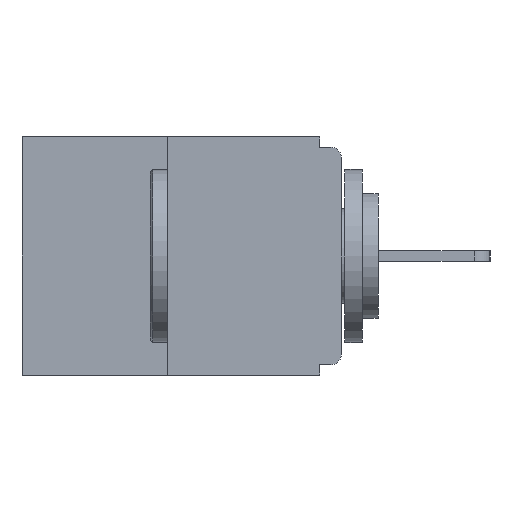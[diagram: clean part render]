
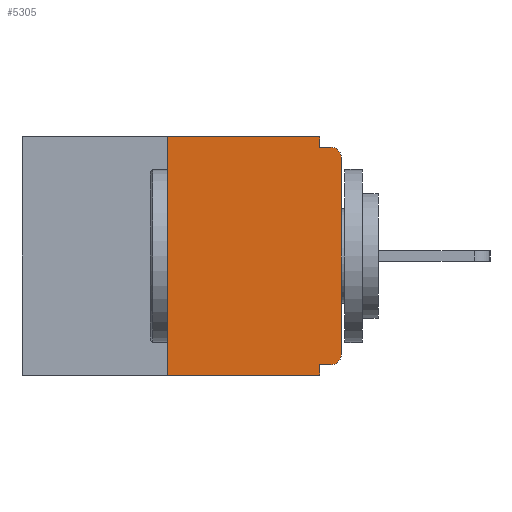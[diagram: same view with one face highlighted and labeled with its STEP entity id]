
A CAD part, left-side view. The second image highlights one B-rep face of the part: STEP entity #5305.
In plain terms, the highlighted planar face has unit normal (-1, 0, 0).
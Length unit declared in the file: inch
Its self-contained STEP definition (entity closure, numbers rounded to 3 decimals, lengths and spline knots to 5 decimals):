
#21 = EDGE_CURVE ( 'NONE', #17906, #2304, #659, .T. ) ;
#180 = ORIENTED_EDGE ( 'NONE', *, *, #4818, .T. ) ;
#387 = CARTESIAN_POINT ( 'NONE',  ( 0., 0.46, 0. ) ) ;
#618 = VECTOR ( 'NONE', #17796, 39.37008 ) ;
#659 = LINE ( 'NONE', #6343, #618 ) ;
#941 = EDGE_LOOP ( 'NONE', ( #14344, #11404, #3829, #10271, #18265, #13380, #5420, #180, #15805, #8281 ) ) ;
#1195 = DIRECTION ( 'NONE',  ( -1., 0., 0. ) ) ;
#1863 = AXIS2_PLACEMENT_3D ( 'NONE', #5914, #3127, #4519 ) ;
#2304 = VERTEX_POINT ( 'NONE', #2717 ) ;
#2305 = CARTESIAN_POINT ( 'NONE',  ( 0., 0.015, -0.328 ) ) ;
#2473 = AXIS2_PLACEMENT_3D ( 'NONE', #387, #11800, #11610 ) ;
#2684 = CARTESIAN_POINT ( 'NONE',  ( 0., 0.031, -0.015 ) ) ;
#2700 = DIRECTION ( 'NONE',  ( 0., 0., 1. ) ) ;
#2717 = CARTESIAN_POINT ( 'NONE',  ( 0., 0., -0.03 ) ) ;
#3127 = DIRECTION ( 'NONE',  ( -1., 0., 0. ) ) ;
#3203 = LINE ( 'NONE', #14530, #13270 ) ;
#3829 = ORIENTED_EDGE ( 'NONE', *, *, #13297, .T. ) ;
#3944 = LINE ( 'NONE', #6741, #12416 ) ;
#4097 = CARTESIAN_POINT ( 'NONE',  ( 0., 0., -0.328 ) ) ;
#4271 = DIRECTION ( 'NONE',  ( 0., 1., 0. ) ) ;
#4519 = DIRECTION ( 'NONE',  ( 0., 0., -1. ) ) ;
#4671 = CARTESIAN_POINT ( 'NONE',  ( 0., 0.031, -0.343 ) ) ;
#4739 = VERTEX_POINT ( 'NONE', #2305 ) ;
#4770 = CARTESIAN_POINT ( 'NONE',  ( 0., 0.25, 0. ) ) ;
#4818 = EDGE_CURVE ( 'NONE', #2304, #14982, #8431, .T. ) ;
#5305 = ADVANCED_FACE ( 'NONE', ( #7473 ), #8697, .F. ) ;
#5420 = ORIENTED_EDGE ( 'NONE', *, *, #21, .T. ) ;
#5493 = LINE ( 'NONE', #4097, #14972 ) ;
#5914 = CARTESIAN_POINT ( 'NONE',  ( 0., 0.015, -0.03 ) ) ;
#6343 = CARTESIAN_POINT ( 'NONE',  ( 0., 0., 0. ) ) ;
#6741 = CARTESIAN_POINT ( 'NONE',  ( 0., 0.46, -0.343 ) ) ;
#6895 = VERTEX_POINT ( 'NONE', #4671 ) ;
#7255 = VECTOR ( 'NONE', #13898, 39.37008 ) ;
#7466 = EDGE_CURVE ( 'NONE', #14918, #6895, #15384, .T. ) ;
#7473 = FACE_OUTER_BOUND ( 'NONE', #941, .T. ) ;
#7769 = EDGE_CURVE ( 'NONE', #10891, #12448, #3203, .T. ) ;
#8281 = ORIENTED_EDGE ( 'NONE', *, *, #18342, .F. ) ;
#8401 = CARTESIAN_POINT ( 'NONE',  ( 0., 0.015, -0.015 ) ) ;
#8431 = CIRCLE ( 'NONE', #1863, 0.015 ) ;
#8697 = PLANE ( 'NONE',  #2473 ) ;
#9292 = CARTESIAN_POINT ( 'NONE',  ( 0., 0., -0.313 ) ) ;
#9453 = CARTESIAN_POINT ( 'NONE',  ( 0., 0.031, 0. ) ) ;
#10120 = DIRECTION ( 'NONE',  ( 0., -1., 0. ) ) ;
#10271 = ORIENTED_EDGE ( 'NONE', *, *, #7466, .F. ) ;
#10651 = CARTESIAN_POINT ( 'NONE',  ( 0., 0.031, 0. ) ) ;
#10891 = VERTEX_POINT ( 'NONE', #4770 ) ;
#10920 = CARTESIAN_POINT ( 'NONE',  ( 0., 0.015, -0.313 ) ) ;
#11103 = VECTOR ( 'NONE', #10120, 39.37008 ) ;
#11116 = EDGE_CURVE ( 'NONE', #17184, #10891, #15722, .T. ) ;
#11152 = VECTOR ( 'NONE', #2700, 39.37008 ) ;
#11404 = ORIENTED_EDGE ( 'NONE', *, *, #11116, .F. ) ;
#11610 = DIRECTION ( 'NONE',  ( 0., 0., -1. ) ) ;
#11616 = DIRECTION ( 'NONE',  ( 0., -1., 0. ) ) ;
#11800 = DIRECTION ( 'NONE',  ( 1., 0., 0. ) ) ;
#12106 = AXIS2_PLACEMENT_3D ( 'NONE', #10920, #1195, #18325 ) ;
#12416 = VECTOR ( 'NONE', #12464, 39.37008 ) ;
#12448 = VERTEX_POINT ( 'NONE', #10651 ) ;
#12464 = DIRECTION ( 'NONE',  ( 0., -1., 0. ) ) ;
#12644 = EDGE_CURVE ( 'NONE', #4739, #17906, #12712, .T. ) ;
#12712 = CIRCLE ( 'NONE', #12106, 0.015 ) ;
#13270 = VECTOR ( 'NONE', #11616, 39.37008 ) ;
#13297 = EDGE_CURVE ( 'NONE', #17184, #6895, #3944, .T. ) ;
#13380 = ORIENTED_EDGE ( 'NONE', *, *, #12644, .T. ) ;
#13482 = LINE ( 'NONE', #9453, #15305 ) ;
#13898 = DIRECTION ( 'NONE',  ( 0., 0., -1. ) ) ;
#13959 = CARTESIAN_POINT ( 'NONE',  ( 0., 0.031, -0.328 ) ) ;
#14344 = ORIENTED_EDGE ( 'NONE', *, *, #7769, .F. ) ;
#14530 = CARTESIAN_POINT ( 'NONE',  ( 0., 0.46, 0. ) ) ;
#14918 = VERTEX_POINT ( 'NONE', #13959 ) ;
#14972 = VECTOR ( 'NONE', #4271, 39.37008 ) ;
#14982 = VERTEX_POINT ( 'NONE', #8401 ) ;
#15305 = VECTOR ( 'NONE', #17900, 39.37008 ) ;
#15373 = EDGE_CURVE ( 'NONE', #4739, #14918, #5493, .T. ) ;
#15384 = LINE ( 'NONE', #17572, #7255 ) ;
#15450 = CARTESIAN_POINT ( 'NONE',  ( 0., 0.25, -0.343 ) ) ;
#15722 = LINE ( 'NONE', #16939, #11152 ) ;
#15805 = ORIENTED_EDGE ( 'NONE', *, *, #16341, .F. ) ;
#15829 = CARTESIAN_POINT ( 'NONE',  ( 0., 0., -0.015 ) ) ;
#16341 = EDGE_CURVE ( 'NONE', #17608, #14982, #17533, .T. ) ;
#16939 = CARTESIAN_POINT ( 'NONE',  ( 0., 0.25, 0. ) ) ;
#17184 = VERTEX_POINT ( 'NONE', #15450 ) ;
#17533 = LINE ( 'NONE', #15829, #11103 ) ;
#17572 = CARTESIAN_POINT ( 'NONE',  ( 0., 0.031, -0.343 ) ) ;
#17608 = VERTEX_POINT ( 'NONE', #2684 ) ;
#17796 = DIRECTION ( 'NONE',  ( 0., 0., 1. ) ) ;
#17900 = DIRECTION ( 'NONE',  ( 0., 0., -1. ) ) ;
#17906 = VERTEX_POINT ( 'NONE', #9292 ) ;
#18265 = ORIENTED_EDGE ( 'NONE', *, *, #15373, .F. ) ;
#18325 = DIRECTION ( 'NONE',  ( 0., 0., -1. ) ) ;
#18342 = EDGE_CURVE ( 'NONE', #12448, #17608, #13482, .T. ) ;
